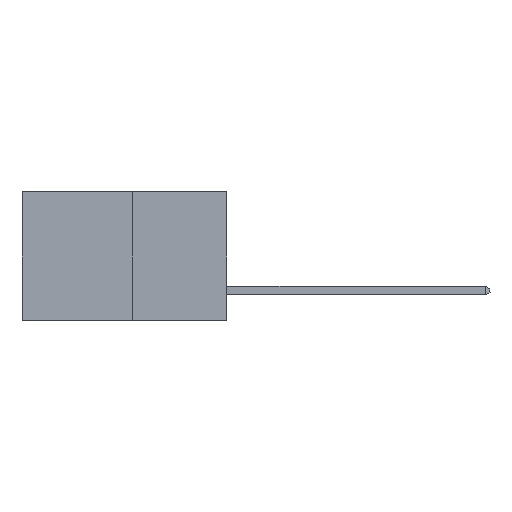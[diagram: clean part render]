
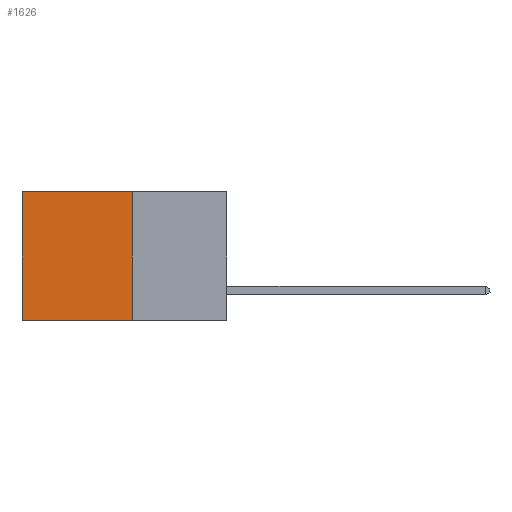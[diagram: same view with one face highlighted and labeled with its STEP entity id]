
A CAD part, left-side view. The second image highlights one B-rep face of the part: STEP entity #1626.
In plain terms, the highlighted planar face has unit normal (-1, 0, 0).
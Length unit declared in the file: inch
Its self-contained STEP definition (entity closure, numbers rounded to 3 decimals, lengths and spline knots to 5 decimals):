
#1049 = CARTESIAN_POINT ( 'NONE',  ( 0.277, 0.27, 0. ) ) ;
#1088 = LINE ( 'NONE', #12430, #9632 ) ;
#1626 = ADVANCED_FACE ( 'NONE', ( #5662 ), #4172, .F. ) ;
#1891 = CARTESIAN_POINT ( 'NONE',  ( 0.277, 0.59, 0. ) ) ;
#2232 = VERTEX_POINT ( 'NONE', #1891 ) ;
#2687 = VERTEX_POINT ( 'NONE', #11027 ) ;
#3708 = DIRECTION ( 'NONE',  ( 0., 0., -1. ) ) ;
#3753 = CARTESIAN_POINT ( 'NONE',  ( 0.277, 0.59, -0.37 ) ) ;
#3864 = ORIENTED_EDGE ( 'NONE', *, *, #12854, .F. ) ;
#4172 = PLANE ( 'NONE',  #10433 ) ;
#4212 = VECTOR ( 'NONE', #3708, 39.37008 ) ;
#4849 = DIRECTION ( 'NONE',  ( 0., 1., 0. ) ) ;
#4908 = ORIENTED_EDGE ( 'NONE', *, *, #10348, .T. ) ;
#5662 = FACE_OUTER_BOUND ( 'NONE', #10477, .T. ) ;
#5746 = EDGE_CURVE ( 'NONE', #2232, #2687, #7500, .T. ) ;
#6080 = VECTOR ( 'NONE', #10961, 39.37008 ) ;
#6384 = CARTESIAN_POINT ( 'NONE',  ( 0.277, 0.27, -0.37 ) ) ;
#7500 = LINE ( 'NONE', #3753, #4212 ) ;
#7560 = DIRECTION ( 'NONE',  ( 1., 0., 0. ) ) ;
#8142 = ORIENTED_EDGE ( 'NONE', *, *, #5746, .T. ) ;
#8591 = DIRECTION ( 'NONE',  ( 0., 0., -1. ) ) ;
#8746 = VECTOR ( 'NONE', #12075, 39.37008 ) ;
#8996 = LINE ( 'NONE', #14017, #6080 ) ;
#9267 = EDGE_CURVE ( 'NONE', #12775, #2687, #1088, .T. ) ;
#9632 = VECTOR ( 'NONE', #4849, 39.37008 ) ;
#9777 = ORIENTED_EDGE ( 'NONE', *, *, #9267, .F. ) ;
#10348 = EDGE_CURVE ( 'NONE', #10665, #2232, #11918, .T. ) ;
#10433 = AXIS2_PLACEMENT_3D ( 'NONE', #6384, #7560, #8591 ) ;
#10477 = EDGE_LOOP ( 'NONE', ( #8142, #9777, #3864, #4908 ) ) ;
#10665 = VERTEX_POINT ( 'NONE', #11565 ) ;
#10961 = DIRECTION ( 'NONE',  ( 0., 0., -1. ) ) ;
#11027 = CARTESIAN_POINT ( 'NONE',  ( 0.277, 0.59, -0.37 ) ) ;
#11565 = CARTESIAN_POINT ( 'NONE',  ( 0.277, 0.27, 0. ) ) ;
#11918 = LINE ( 'NONE', #1049, #8746 ) ;
#12075 = DIRECTION ( 'NONE',  ( 0., 1., 0. ) ) ;
#12430 = CARTESIAN_POINT ( 'NONE',  ( 0.277, 0.27, -0.37 ) ) ;
#12775 = VERTEX_POINT ( 'NONE', #13200 ) ;
#12854 = EDGE_CURVE ( 'NONE', #10665, #12775, #8996, .T. ) ;
#13200 = CARTESIAN_POINT ( 'NONE',  ( 0.277, 0.27, -0.37 ) ) ;
#14017 = CARTESIAN_POINT ( 'NONE',  ( 0.277, 0.27, -0.37 ) ) ;
